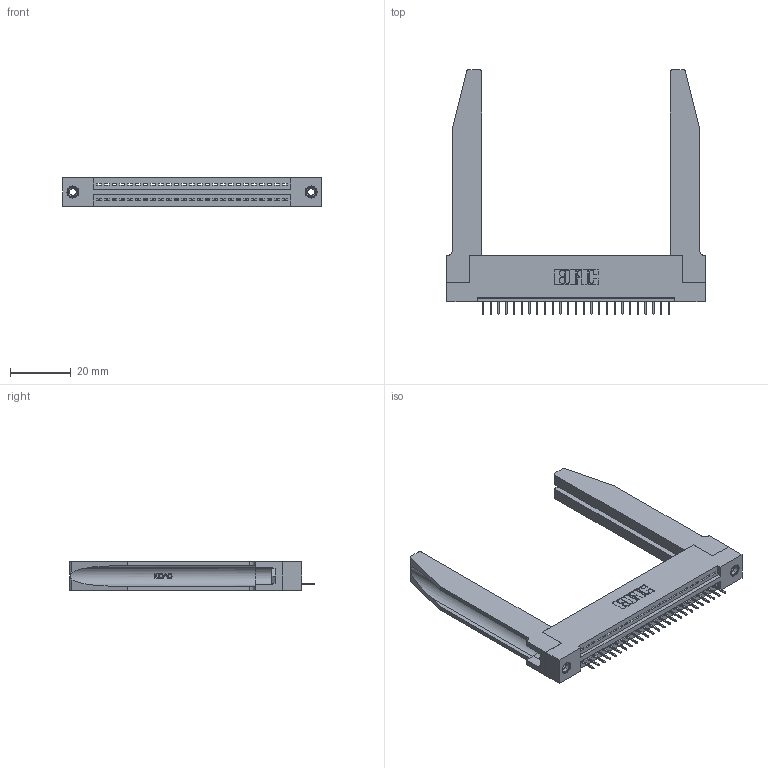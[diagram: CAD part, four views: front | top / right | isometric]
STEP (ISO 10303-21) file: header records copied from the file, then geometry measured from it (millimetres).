
FILE_DESCRIPTION (( 'STEP AP203' ), '1' );
FILE_NAME ('395-025-524-178.STEP', '2019-10-18T07:36:52', ( '' ), ( '' ), 'SwSTEP 2.0', 'SolidWorks 2016', '' );
FILE_SCHEMA (( 'CONFIG_CONTROL_DESIGN' ));
Length unit declared in the file: inch
Products named in the file (5): 345-220-078_345-220-078; 345-292-001_345-293-124; 345-250-001_345-250-001-102; 395-025-524-178; 345 Part_Flush Mounting Lugs - 0.156 Dia-TH
Assembly tree (30 placements, depth 2):
  395-025-524-178
    345 Part_Flush Mounting Lugs - 0.156 Dia-TH
    345-292-001_345-293-124  x25
    345-250-001_345-250-001-102  x2
    345-220-078_345-220-078  x2
Bounding box: 84.73 x 80.31 x 9.4 mm (x, y, z)
Volume: 15580.6 mm3; surface area: 16677.8 mm2
Topology: 30 solids, 30 shells, 1910 faces, 5449 edges, 3522 vertices
Faces by surface type: plane 1372, cylinder 486, bspline 36, cone 12, torus 4
Entity records: 25918 total; most frequent: CARTESIAN_POINT 5386, ORIENTED_EDGE 4242, DIRECTION 3737, EDGE_CURVE 2121, LINE 1799, VECTOR 1799, VERTEX_POINT 1404, AXIS2_PLACEMENT_3D 969
